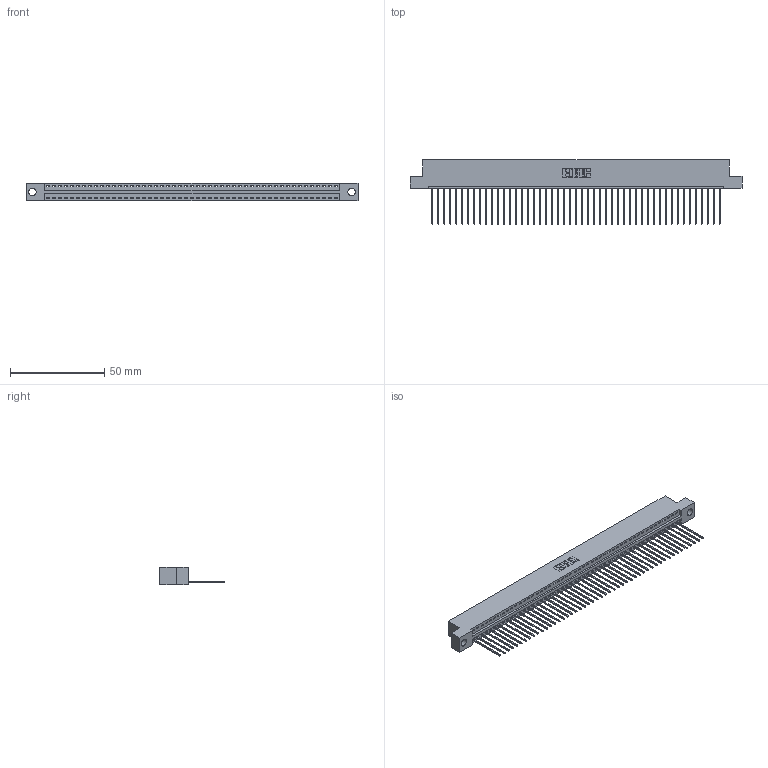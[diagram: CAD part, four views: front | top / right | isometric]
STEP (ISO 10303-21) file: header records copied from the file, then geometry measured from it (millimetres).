
FILE_DESCRIPTION (( 'STEP AP203' ), '1' );
FILE_NAME ('346-049-541-104.STEP', '2018-08-25T12:25:15', ( '' ), ( '' ), 'SwSTEP 2.0', 'SolidWorks 2016', '' );
FILE_SCHEMA (( 'CONFIG_CONTROL_DESIGN' ));
Length unit declared in the file: inch
Products named in the file (3): 346 Part_Flush Mounting Lugs - 0.156 Dia-TH; 345-292-001_345-293-141; 346-049-541-104
Assembly tree (50 placements, depth 2):
  346-049-541-104
    346 Part_Flush Mounting Lugs - 0.156 Dia-TH
    345-292-001_345-293-141  x49
Bounding box: 176.15 x 34.29 x 9.4 mm (x, y, z)
Volume: 16983.4 mm3; surface area: 22073.5 mm2
Topology: 50 solids, 50 shells, 2964 faces, 8953 edges, 5902 vertices
Faces by surface type: plane 2036, cylinder 928
Entity records: 29489 total; most frequent: CARTESIAN_POINT 5059, ORIENTED_EDGE 5042, DIRECTION 4455, EDGE_CURVE 2521, LINE 2193, VECTOR 2193, VERTEX_POINT 1678, AXIS2_PLACEMENT_3D 1131
